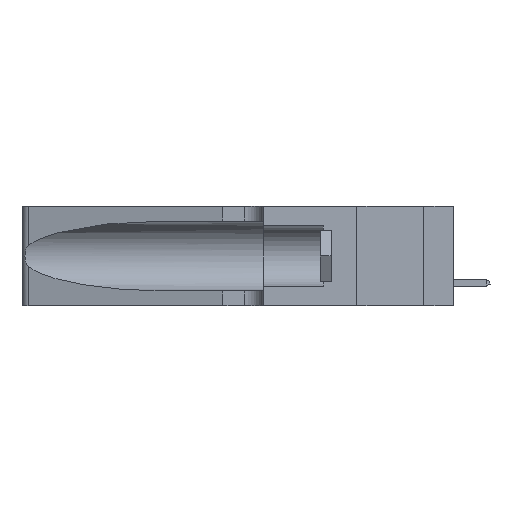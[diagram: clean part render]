
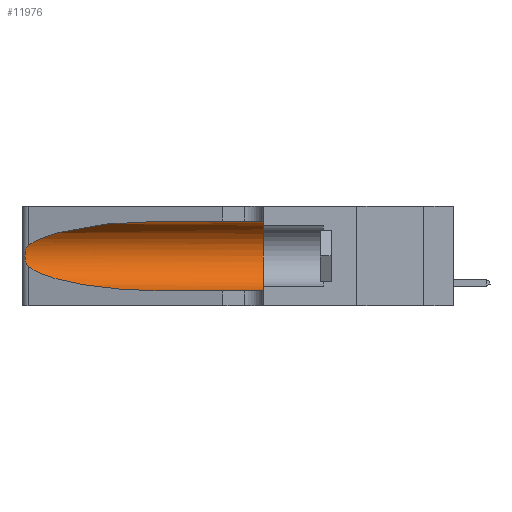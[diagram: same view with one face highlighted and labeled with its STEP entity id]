
A CAD part, left-side view. The second image highlights one B-rep face of the part: STEP entity #11976.
In plain terms, the highlighted cylindrical face has radius 3.308 mm (diameter 6.617 mm), a partial arc.
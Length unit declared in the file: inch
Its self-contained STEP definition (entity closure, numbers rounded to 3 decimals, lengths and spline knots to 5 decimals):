
#1066 = CARTESIAN_POINT ( 'NONE',  ( 0.2373, 1.15595, 0.08982 ) ) ;
#1491 = CARTESIAN_POINT ( 'NONE',  ( 0.25555, 1.22994, 0.2215 ) ) ;
#2211 = DIRECTION ( 'NONE',  ( 0., -1., 0. ) ) ;
#2768 = CARTESIAN_POINT ( 'NONE',  ( 0.18966, 0.96281, 0.31525 ) ) ;
#3187 = LINE ( 'NONE', #46917, #50063 ) ;
#4079 = VERTEX_POINT ( 'NONE', #45311 ) ;
#4088 = VERTEX_POINT ( 'NONE', #46356 ) ;
#6243 = VECTOR ( 'NONE', #42451, 39.37008 ) ;
#6389 = CARTESIAN_POINT ( 'NONE',  ( 0.1305, 1.61858, 0.31525 ) ) ;
#6681 = ORIENTED_EDGE ( 'NONE', *, *, #40351, .T. ) ;
#6693 = CARTESIAN_POINT ( 'NONE',  ( 0.25487, 1.22718, 0.22369 ) ) ;
#7722 = DIRECTION ( 'NONE',  ( 0., 0., 1. ) ) ;
#8079 = ORIENTED_EDGE ( 'NONE', *, *, #8162, .T. ) ;
#8162 = EDGE_CURVE ( 'NONE', #15020, #20939, #3187, .T. ) ;
#11976 = ADVANCED_FACE ( 'NONE', ( #31947 ), #14192, .F. ) ;
#12870 = CARTESIAN_POINT ( 'NONE',  ( 0.1305, 0.35, 0.05475 ) ) ;
#12995 = CARTESIAN_POINT ( 'NONE',  ( 0.1305, 0.72297, 0.05475 ) ) ;
#13524 = EDGE_LOOP ( 'NONE', ( #6681, #35889, #16917, #8079, #46635, #48381 ) ) ;
#13663 =( BOUNDED_CURVE ( )  B_SPLINE_CURVE ( 3, ( #29353, #1066, #46000, #21554 ),
 .UNSPECIFIED., .F., .F. ) 
 B_SPLINE_CURVE_WITH_KNOTS ( ( 4, 4 ),
 ( 3.44316, 4.71239 ),
 .UNSPECIFIED. ) 
 CURVE ( )  GEOMETRIC_REPRESENTATION_ITEM ( )  RATIONAL_B_SPLINE_CURVE ( ( 1., 0.87, 0.87, 1. ) ) 
 REPRESENTATION_ITEM ( '' )  );
#13686 = CARTESIAN_POINT ( 'NONE',  ( 0.26018, 1.23835, 0.19895 ) ) ;
#14192 = CYLINDRICAL_SURFACE ( 'NONE', #24753, 0.13025 ) ;
#15020 = VERTEX_POINT ( 'NONE', #12995 ) ;
#16917 = ORIENTED_EDGE ( 'NONE', *, *, #47478, .T. ) ;
#17007 = LINE ( 'NONE', #6389, #6243 ) ;
#20939 = VERTEX_POINT ( 'NONE', #12870 ) ;
#21554 = CARTESIAN_POINT ( 'NONE',  ( 0.1305, 0.72297, 0.05475 ) ) ;
#21647 = CARTESIAN_POINT ( 'NONE',  ( 0.25787, 1.23484, 0.2124 ) ) ;
#22343 = CARTESIAN_POINT ( 'NONE',  ( 0.25639, 1.23186, 0.15144 ) ) ;
#22874 = DIRECTION ( 'NONE',  ( 0., 0., -1. ) ) ;
#23859 = DIRECTION ( 'NONE',  ( 0., -1., 0. ) ) ;
#24116 = DIRECTION ( 'NONE',  ( 0., 1., 0. ) ) ;
#24633 = CARTESIAN_POINT ( 'NONE',  ( 0.1305, 0.35, 0.185 ) ) ;
#24753 = AXIS2_PLACEMENT_3D ( 'NONE', #41837, #2211, #22874 ) ;
#25719 = CARTESIAN_POINT ( 'NONE',  ( 0.26075, 1.23896, 0.19203 ) ) ;
#25886 = CARTESIAN_POINT ( 'NONE',  ( 0.25789, 1.23486, 0.15765 ) ) ;
#26814 = CARTESIAN_POINT ( 'NONE',  ( 0.2373, 1.15595, 0.28018 ) ) ;
#26977 = CARTESIAN_POINT ( 'NONE',  ( 0.1305, 0.72297, 0.31525 ) ) ;
#29353 = CARTESIAN_POINT ( 'NONE',  ( 0.25487, 1.22718, 0.14631 ) ) ;
#29785 = CARTESIAN_POINT ( 'NONE',  ( 0.25856, 1.23593, 0.16098 ) ) ;
#29958 = CARTESIAN_POINT ( 'NONE',  ( 0.25555, 1.22993, 0.14849 ) ) ;
#30868 =( BOUNDED_CURVE ( )  B_SPLINE_CURVE ( 3, ( #26977, #2768, #26814, #6693 ),
 .UNSPECIFIED., .F., .F. ) 
 B_SPLINE_CURVE_WITH_KNOTS ( ( 4, 4 ),
 ( 1.5708, 2.84003 ),
 .UNSPECIFIED. ) 
 CURVE ( )  GEOMETRIC_REPRESENTATION_ITEM ( )  RATIONAL_B_SPLINE_CURVE ( ( 1., 0.87, 0.87, 1. ) ) 
 REPRESENTATION_ITEM ( '' )  );
#31370 = CARTESIAN_POINT ( 'NONE',  ( 0.25487, 1.22718, 0.22369 ) ) ;
#31947 = FACE_OUTER_BOUND ( 'NONE', #13524, .T. ) ;
#33381 = AXIS2_PLACEMENT_3D ( 'NONE', #24633, #24116, #7722 ) ;
#35889 = ORIENTED_EDGE ( 'NONE', *, *, #40948, .T. ) ;
#36409 = B_SPLINE_CURVE_WITH_KNOTS ( 'NONE', 3,
 ( #38276, #1491, #38442, #21647, #37762, #13686, #25719, #42517, #46607, #29785, #25886, #22343, #29958, #50696 ),
 .UNSPECIFIED., .F., .F.,
 ( 4, 2, 2, 2, 2, 2, 4 ),
 ( 0., 0.00027, 0.00053, 0.00107, 0.0016, 0.00187, 0.00214 ),
 .UNSPECIFIED. ) ;
#37762 = CARTESIAN_POINT ( 'NONE',  ( 0.25854, 1.2359, 0.20912 ) ) ;
#38276 = CARTESIAN_POINT ( 'NONE',  ( 0.25487, 1.22718, 0.22369 ) ) ;
#38442 = CARTESIAN_POINT ( 'NONE',  ( 0.25639, 1.23184, 0.21858 ) ) ;
#40351 = EDGE_CURVE ( 'NONE', #4079, #44373, #30868, .T. ) ;
#40948 = EDGE_CURVE ( 'NONE', #44373, #46927, #36409, .T. ) ;
#41559 = EDGE_CURVE ( 'NONE', #4079, #4088, #17007, .T. ) ;
#41837 = CARTESIAN_POINT ( 'NONE',  ( 0.1305, 1.61858, 0.185 ) ) ;
#42451 = DIRECTION ( 'NONE',  ( 0., -1., 0. ) ) ;
#42517 = CARTESIAN_POINT ( 'NONE',  ( 0.26075, 1.23896, 0.178 ) ) ;
#44373 = VERTEX_POINT ( 'NONE', #31370 ) ;
#45311 = CARTESIAN_POINT ( 'NONE',  ( 0.1305, 0.72297, 0.31525 ) ) ;
#46000 = CARTESIAN_POINT ( 'NONE',  ( 0.18966, 0.96281, 0.05475 ) ) ;
#46356 = CARTESIAN_POINT ( 'NONE',  ( 0.1305, 0.35, 0.31525 ) ) ;
#46607 = CARTESIAN_POINT ( 'NONE',  ( 0.26017, 1.23833, 0.17102 ) ) ;
#46635 = ORIENTED_EDGE ( 'NONE', *, *, #46764, .F. ) ;
#46764 = EDGE_CURVE ( 'NONE', #4088, #20939, #50456, .T. ) ;
#46917 = CARTESIAN_POINT ( 'NONE',  ( 0.1305, 1.61858, 0.05475 ) ) ;
#46927 = VERTEX_POINT ( 'NONE', #49631 ) ;
#47478 = EDGE_CURVE ( 'NONE', #46927, #15020, #13663, .T. ) ;
#48381 = ORIENTED_EDGE ( 'NONE', *, *, #41559, .F. ) ;
#49631 = CARTESIAN_POINT ( 'NONE',  ( 0.25487, 1.22718, 0.14631 ) ) ;
#50063 = VECTOR ( 'NONE', #23859, 39.37008 ) ;
#50456 = CIRCLE ( 'NONE', #33381, 0.13025 ) ;
#50696 = CARTESIAN_POINT ( 'NONE',  ( 0.25487, 1.22718, 0.14631 ) ) ;
